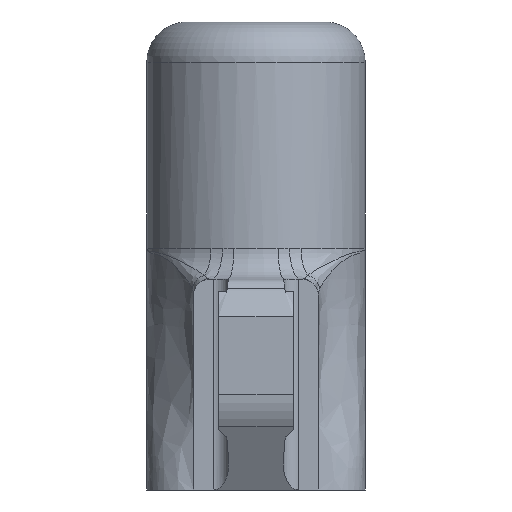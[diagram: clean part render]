
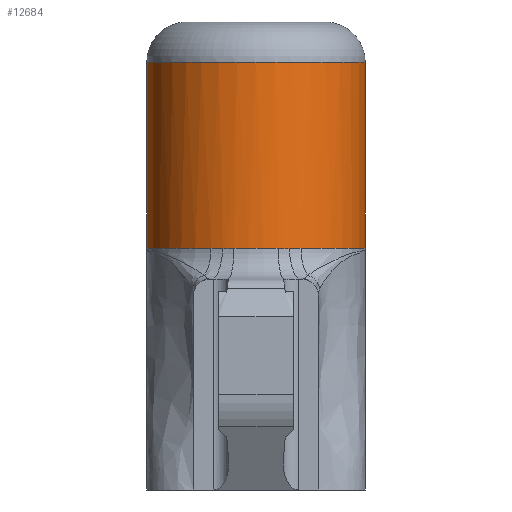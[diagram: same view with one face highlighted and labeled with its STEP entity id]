
A CAD part, front view. The second image highlights one B-rep face of the part: STEP entity #12684.
In plain terms, the highlighted cylindrical face has radius 17.5 mm (diameter 35 mm), a partial arc.
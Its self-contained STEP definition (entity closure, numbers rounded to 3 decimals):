
#50 = CIRCLE ( 'NONE', #1825, 17.5 ) ;
#166 = ORIENTED_EDGE ( 'NONE', *, *, #11505, .T. ) ;
#404 = CARTESIAN_POINT ( 'NONE',  ( -4.738, -16.847, 38.664 ) ) ;
#625 = ORIENTED_EDGE ( 'NONE', *, *, #8825, .T. ) ;
#906 = EDGE_CURVE ( 'NONE', #3142, #4823, #50, .T. ) ;
#1117 = VERTEX_POINT ( 'NONE', #4955 ) ;
#1488 = CARTESIAN_POINT ( 'NONE',  ( -17.5, 0., 75. ) ) ;
#1521 = CARTESIAN_POINT ( 'NONE',  ( -4.142, -17.006, 38.723 ) ) ;
#1522 = CARTESIAN_POINT ( 'NONE',  ( 0., 0., 68.53 ) ) ;
#1524 = CARTESIAN_POINT ( 'NONE',  ( 5.972, -16.463, 38.722 ) ) ;
#1554 = CARTESIAN_POINT ( 'NONE',  ( 17.5, 0., 68.53 ) ) ;
#1625 = CARTESIAN_POINT ( 'NONE',  ( 7.213, -15.944, 38.759 ) ) ;
#1788 = CARTESIAN_POINT ( 'NONE',  ( -17.5, 0., 68.53 ) ) ;
#1823 = DIRECTION ( 'NONE',  ( 0., 0., -1. ) ) ;
#1825 = AXIS2_PLACEMENT_3D ( 'NONE', #5941, #13696, #7060 ) ;
#2076 = VERTEX_POINT ( 'NONE', #14167 ) ;
#2145 = VERTEX_POINT ( 'NONE', #6238 ) ;
#2236 = EDGE_LOOP ( 'NONE', ( #3911, #3447, #4024, #12073, #5904, #13915, #625, #166, #4398, #12717 ) ) ;
#2298 = CIRCLE ( 'NONE', #5876, 17.5 ) ;
#2501 = EDGE_CURVE ( 'NONE', #2145, #8522, #10538, .T. ) ;
#2534 = CARTESIAN_POINT ( 'NONE',  ( -5.332, -16.668, 38.672 ) ) ;
#2636 = CARTESIAN_POINT ( 'NONE',  ( -3.538, -17.139, 38.759 ) ) ;
#2637 = DIRECTION ( 'NONE',  ( 1., 0., 0. ) ) ;
#2639 = CARTESIAN_POINT ( 'NONE',  ( 5.332, -16.668, 38.672 ) ) ;
#2915 = CARTESIAN_POINT ( 'NONE',  ( 17.5, 0., 38.759 ) ) ;
#2984 = EDGE_CURVE ( 'NONE', #6994, #8522, #11048, .T. ) ;
#3142 = VERTEX_POINT ( 'NONE', #6066 ) ;
#3146 = VECTOR ( 'NONE', #9241, 1000. ) ;
#3447 = ORIENTED_EDGE ( 'NONE', *, *, #12294, .T. ) ;
#3911 = ORIENTED_EDGE ( 'NONE', *, *, #2984, .F. ) ;
#4024 = ORIENTED_EDGE ( 'NONE', *, *, #5820, .T. ) ;
#4058 = CARTESIAN_POINT ( 'NONE',  ( -5.332, -16.668, 38.672 ) ) ;
#4243 = CARTESIAN_POINT ( 'NONE',  ( 4.142, -17.006, 38.723 ) ) ;
#4331 = EDGE_CURVE ( 'NONE', #4823, #1117, #5482, .T. ) ;
#4346 = DIRECTION ( 'NONE',  ( 0., 0., -1. ) ) ;
#4398 = ORIENTED_EDGE ( 'NONE', *, *, #13441, .T. ) ;
#4689 = CARTESIAN_POINT ( 'NONE',  ( -3.538, -17.139, 38.759 ) ) ;
#4823 = VERTEX_POINT ( 'NONE', #10296 ) ;
#4955 = CARTESIAN_POINT ( 'NONE',  ( -5.332, -16.668, 38.672 ) ) ;
#5346 = CARTESIAN_POINT ( 'NONE',  ( 4.738, -16.847, 38.664 ) ) ;
#5482 = B_SPLINE_CURVE_WITH_KNOTS ( 'NONE', 3,
 ( #13980, #9587, #10698, #4058 ),
 .UNSPECIFIED., .F., .F.,
 ( 4, 4 ),
 ( 0., 0.002 ),
 .UNSPECIFIED. ) ;
#5531 = DIRECTION ( 'NONE',  ( 0., 0., 1. ) ) ;
#5820 = EDGE_CURVE ( 'NONE', #13920, #3142, #9024, .T. ) ;
#5876 = AXIS2_PLACEMENT_3D ( 'NONE', #1522, #9278, #2637 ) ;
#5904 = ORIENTED_EDGE ( 'NONE', *, *, #4331, .T. ) ;
#5941 = CARTESIAN_POINT ( 'NONE',  ( 0., 0., 38.759 ) ) ;
#5980 = DIRECTION ( 'NONE',  ( 0., 0., 1. ) ) ;
#6066 = CARTESIAN_POINT ( 'NONE',  ( -17.5, 0., 38.759 ) ) ;
#6238 = CARTESIAN_POINT ( 'NONE',  ( 7.213, -15.944, 38.759 ) ) ;
#6272 = EDGE_CURVE ( 'NONE', #1117, #6594, #7784, .T. ) ;
#6321 = CARTESIAN_POINT ( 'NONE',  ( 5.332, -16.668, 38.672 ) ) ;
#6457 = CARTESIAN_POINT ( 'NONE',  ( 5.184, -16.715, 38.66 ) ) ;
#6594 = VERTEX_POINT ( 'NONE', #4689 ) ;
#6994 = VERTEX_POINT ( 'NONE', #1554 ) ;
#7035 = CARTESIAN_POINT ( 'NONE',  ( -5.035, -16.761, 38.655 ) ) ;
#7060 = DIRECTION ( 'NONE',  ( -1., 0., 0. ) ) ;
#7523 = FACE_OUTER_BOUND ( 'NONE', #2236, .T. ) ;
#7784 = B_SPLINE_CURVE_WITH_KNOTS ( 'NONE', 3,
 ( #2534, #11393, #7035, #404, #8144, #1521, #9276, #2636 ),
 .UNSPECIFIED., .F., .F.,
 ( 4, 2, 2, 4 ),
 ( 0., 0., 0.001, 0.002 ),
 .UNSPECIFIED. ) ;
#8144 = CARTESIAN_POINT ( 'NONE',  ( -4.589, -16.888, 38.677 ) ) ;
#8253 = CARTESIAN_POINT ( 'NONE',  ( 6.599, -16.222, 38.759 ) ) ;
#8459 = VECTOR ( 'NONE', #4346, 1000. ) ;
#8522 = VERTEX_POINT ( 'NONE', #2915 ) ;
#8825 = EDGE_CURVE ( 'NONE', #6594, #2076, #12364, .T. ) ;
#8881 = B_SPLINE_CURVE_WITH_KNOTS ( 'NONE', 3,
 ( #9773, #10880, #4243, #11985, #5346, #13093, #6457, #14208 ),
 .UNSPECIFIED., .F., .F.,
 ( 4, 2, 2, 4 ),
 ( 0., 0.001, 0.001, 0.002 ),
 .UNSPECIFIED. ) ;
#9024 = LINE ( 'NONE', #1488, #3146 ) ;
#9241 = DIRECTION ( 'NONE',  ( 0., 0., -1. ) ) ;
#9276 = CARTESIAN_POINT ( 'NONE',  ( -3.842, -17.076, 38.759 ) ) ;
#9278 = DIRECTION ( 'NONE',  ( 0., 0., -1. ) ) ;
#9578 = CARTESIAN_POINT ( 'NONE',  ( 0., 0., 75. ) ) ;
#9587 = CARTESIAN_POINT ( 'NONE',  ( -6.599, -16.222, 38.759 ) ) ;
#9630 = DIRECTION ( 'NONE',  ( -1., 0., 0. ) ) ;
#9773 = CARTESIAN_POINT ( 'NONE',  ( 3.538, -17.139, 38.759 ) ) ;
#9909 = AXIS2_PLACEMENT_3D ( 'NONE', #12609, #5980, #13734 ) ;
#9966 = CARTESIAN_POINT ( 'NONE',  ( 17.5, 0., 75. ) ) ;
#10119 = AXIS2_PLACEMENT_3D ( 'NONE', #12167, #5531, #13277 ) ;
#10296 = CARTESIAN_POINT ( 'NONE',  ( -7.213, -15.944, 38.759 ) ) ;
#10538 = CIRCLE ( 'NONE', #9909, 17.5 ) ;
#10698 = CARTESIAN_POINT ( 'NONE',  ( -5.972, -16.463, 38.722 ) ) ;
#10880 = CARTESIAN_POINT ( 'NONE',  ( 3.842, -17.076, 38.759 ) ) ;
#11048 = LINE ( 'NONE', #9966, #8459 ) ;
#11393 = CARTESIAN_POINT ( 'NONE',  ( -5.184, -16.715, 38.66 ) ) ;
#11505 = EDGE_CURVE ( 'NONE', #2076, #12710, #8881, .T. ) ;
#11985 = CARTESIAN_POINT ( 'NONE',  ( 4.589, -16.888, 38.677 ) ) ;
#12073 = ORIENTED_EDGE ( 'NONE', *, *, #906, .T. ) ;
#12081 = B_SPLINE_CURVE_WITH_KNOTS ( 'NONE', 3,
 ( #2639, #1524, #8253, #1625 ),
 .UNSPECIFIED., .F., .F.,
 ( 4, 4 ),
 ( 0., 0.002 ),
 .UNSPECIFIED. ) ;
#12167 = CARTESIAN_POINT ( 'NONE',  ( 0., 0., 38.759 ) ) ;
#12294 = EDGE_CURVE ( 'NONE', #6994, #13920, #2298, .T. ) ;
#12364 = CIRCLE ( 'NONE', #10119, 17.5 ) ;
#12609 = CARTESIAN_POINT ( 'NONE',  ( 0., 0., 38.759 ) ) ;
#12684 = ADVANCED_FACE ( 'NONE', ( #7523 ), #13056, .T. ) ;
#12710 = VERTEX_POINT ( 'NONE', #6321 ) ;
#12717 = ORIENTED_EDGE ( 'NONE', *, *, #2501, .T. ) ;
#13056 = CYLINDRICAL_SURFACE ( 'NONE', #13302, 17.5 ) ;
#13093 = CARTESIAN_POINT ( 'NONE',  ( 5.035, -16.761, 38.655 ) ) ;
#13277 = DIRECTION ( 'NONE',  ( -1., 0., 0. ) ) ;
#13302 = AXIS2_PLACEMENT_3D ( 'NONE', #9578, #1823, #9630 ) ;
#13441 = EDGE_CURVE ( 'NONE', #12710, #2145, #12081, .T. ) ;
#13696 = DIRECTION ( 'NONE',  ( 0., 0., 1. ) ) ;
#13734 = DIRECTION ( 'NONE',  ( -1., 0., 0. ) ) ;
#13915 = ORIENTED_EDGE ( 'NONE', *, *, #6272, .T. ) ;
#13920 = VERTEX_POINT ( 'NONE', #1788 ) ;
#13980 = CARTESIAN_POINT ( 'NONE',  ( -7.213, -15.944, 38.759 ) ) ;
#14167 = CARTESIAN_POINT ( 'NONE',  ( 3.538, -17.139, 38.759 ) ) ;
#14208 = CARTESIAN_POINT ( 'NONE',  ( 5.332, -16.668, 38.672 ) ) ;
